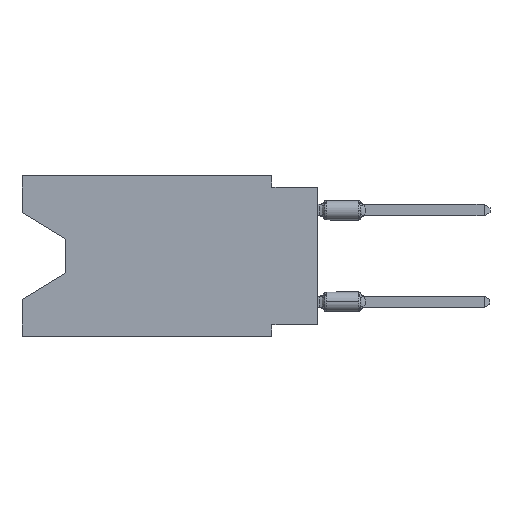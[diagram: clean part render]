
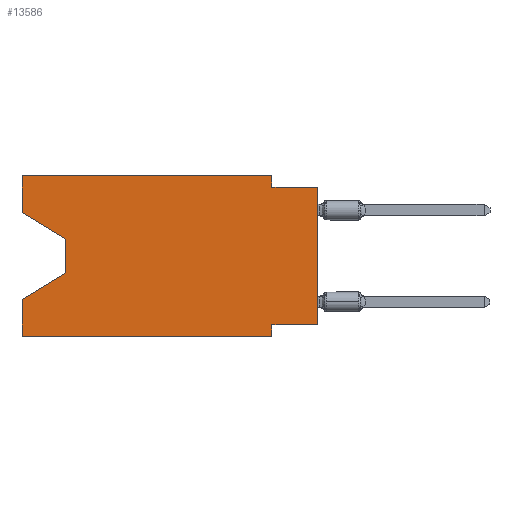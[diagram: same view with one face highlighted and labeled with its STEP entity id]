
A CAD part, left-side view. The second image highlights one B-rep face of the part: STEP entity #13586.
In plain terms, the highlighted planar face has unit normal (-1, 0, 0).
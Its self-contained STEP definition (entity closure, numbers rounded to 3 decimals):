
#43 = VERTEX_POINT ( 'NONE', #5842 ) ;
#48 = DIRECTION ( 'NONE',  ( 0., 0., 1. ) ) ;
#241 = CARTESIAN_POINT ( 'NONE',  ( 0., 2.54, -0.635 ) ) ;
#380 = VECTOR ( 'NONE', #11829, 1000. ) ;
#426 = CARTESIAN_POINT ( 'NONE',  ( 0., 0., -8.255 ) ) ;
#474 = EDGE_CURVE ( 'NONE', #11368, #16184, #8024, .T. ) ;
#653 = DIRECTION ( 'NONE',  ( 0., -1., 0. ) ) ;
#946 = CARTESIAN_POINT ( 'NONE',  ( 0., 2.54, -8.255 ) ) ;
#982 = CARTESIAN_POINT ( 'NONE',  ( 0., 16.383, 0. ) ) ;
#1346 = PLANE ( 'NONE',  #4279 ) ;
#1744 = LINE ( 'NONE', #7595, #12740 ) ;
#1861 = CARTESIAN_POINT ( 'NONE',  ( 0., 16.383, -8.89 ) ) ;
#1986 = LINE ( 'NONE', #13140, #380 ) ;
#2084 = DIRECTION ( 'NONE',  ( 0., 0., 1. ) ) ;
#2108 = CARTESIAN_POINT ( 'NONE',  ( 0., 2.54, 0. ) ) ;
#2224 = CARTESIAN_POINT ( 'NONE',  ( 0., 16.383, -8.89 ) ) ;
#2281 = VECTOR ( 'NONE', #18322, 1000. ) ;
#2501 = ORIENTED_EDGE ( 'NONE', *, *, #15400, .F. ) ;
#2663 = VERTEX_POINT ( 'NONE', #426 ) ;
#2858 = VECTOR ( 'NONE', #16302, 1000. ) ;
#2862 = EDGE_CURVE ( 'NONE', #5707, #16420, #9345, .T. ) ;
#2960 = CARTESIAN_POINT ( 'NONE',  ( 0., 16.383, -2.038 ) ) ;
#3248 = EDGE_CURVE ( 'NONE', #10550, #15878, #7563, .T. ) ;
#3447 = VERTEX_POINT ( 'NONE', #17375 ) ;
#3516 = VECTOR ( 'NONE', #48, 1000. ) ;
#3518 = CARTESIAN_POINT ( 'NONE',  ( 0., 13.97, -3.505 ) ) ;
#3619 = ORIENTED_EDGE ( 'NONE', *, *, #9178, .T. ) ;
#4067 = CARTESIAN_POINT ( 'NONE',  ( 0., 13.97, -3.505 ) ) ;
#4155 = ORIENTED_EDGE ( 'NONE', *, *, #17884, .T. ) ;
#4279 = AXIS2_PLACEMENT_3D ( 'NONE', #12594, #7189, #7271 ) ;
#4554 = DIRECTION ( 'NONE',  ( 0., -1., 0. ) ) ;
#4651 = CARTESIAN_POINT ( 'NONE',  ( 0., 16.383, 0. ) ) ;
#4839 = LINE ( 'NONE', #4651, #13966 ) ;
#5613 = VERTEX_POINT ( 'NONE', #12944 ) ;
#5678 = CARTESIAN_POINT ( 'NONE',  ( 0., 13.97, -5.385 ) ) ;
#5707 = VERTEX_POINT ( 'NONE', #10988 ) ;
#5842 = CARTESIAN_POINT ( 'NONE',  ( 0., 0., -0.635 ) ) ;
#6115 = VECTOR ( 'NONE', #8642, 1000. ) ;
#6698 = ORIENTED_EDGE ( 'NONE', *, *, #11343, .F. ) ;
#7189 = DIRECTION ( 'NONE',  ( 1., 0., 0. ) ) ;
#7271 = DIRECTION ( 'NONE',  ( 0., 0., -1. ) ) ;
#7288 = CARTESIAN_POINT ( 'NONE',  ( 0., 0., 0. ) ) ;
#7563 = LINE ( 'NONE', #17420, #17422 ) ;
#7582 = DIRECTION ( 'NONE',  ( 0., 0., -1. ) ) ;
#7595 = CARTESIAN_POINT ( 'NONE',  ( 0., 0., -0.635 ) ) ;
#7803 = ORIENTED_EDGE ( 'NONE', *, *, #15040, .F. ) ;
#8024 = LINE ( 'NONE', #13697, #2858 ) ;
#8642 = DIRECTION ( 'NONE',  ( 0., -0.855, -0.519 ) ) ;
#8944 = EDGE_LOOP ( 'NONE', ( #4155, #11613, #11654, #17715, #15608, #7803, #2501, #3619, #12137, #17951, #6698, #16190 ) ) ;
#9178 = EDGE_CURVE ( 'NONE', #2663, #43, #15581, .T. ) ;
#9345 = LINE ( 'NONE', #2108, #9988 ) ;
#9988 = VECTOR ( 'NONE', #7582, 1000. ) ;
#10150 = CARTESIAN_POINT ( 'NONE',  ( 0., 16.383, -6.852 ) ) ;
#10307 = LINE ( 'NONE', #10490, #12962 ) ;
#10490 = CARTESIAN_POINT ( 'NONE',  ( 0., 0., -8.255 ) ) ;
#10535 = EDGE_CURVE ( 'NONE', #16420, #43, #1744, .T. ) ;
#10550 = VERTEX_POINT ( 'NONE', #2960 ) ;
#10564 = LINE ( 'NONE', #3518, #14697 ) ;
#10988 = CARTESIAN_POINT ( 'NONE',  ( 0., 2.54, 0. ) ) ;
#11072 = LINE ( 'NONE', #5678, #2281 ) ;
#11343 = EDGE_CURVE ( 'NONE', #15878, #5707, #4839, .T. ) ;
#11368 = VERTEX_POINT ( 'NONE', #1861 ) ;
#11457 = VERTEX_POINT ( 'NONE', #946 ) ;
#11613 = ORIENTED_EDGE ( 'NONE', *, *, #14179, .T. ) ;
#11654 = ORIENTED_EDGE ( 'NONE', *, *, #17752, .T. ) ;
#11829 = DIRECTION ( 'NONE',  ( 0., 0., -1. ) ) ;
#12086 = VERTEX_POINT ( 'NONE', #4067 ) ;
#12137 = ORIENTED_EDGE ( 'NONE', *, *, #10535, .F. ) ;
#12594 = CARTESIAN_POINT ( 'NONE',  ( 0., 16.383, 0. ) ) ;
#12740 = VECTOR ( 'NONE', #17550, 1000. ) ;
#12825 = CARTESIAN_POINT ( 'NONE',  ( 0., 16.383, -2.038 ) ) ;
#12944 = CARTESIAN_POINT ( 'NONE',  ( 0., 2.54, -8.89 ) ) ;
#12962 = VECTOR ( 'NONE', #15989, 1000. ) ;
#13140 = CARTESIAN_POINT ( 'NONE',  ( 0., 2.54, -8.89 ) ) ;
#13586 = ADVANCED_FACE ( 'NONE', ( #14255 ), #1346, .F. ) ;
#13697 = CARTESIAN_POINT ( 'NONE',  ( 0., 16.383, 0. ) ) ;
#13966 = VECTOR ( 'NONE', #4554, 1000. ) ;
#14179 = EDGE_CURVE ( 'NONE', #12086, #3447, #10564, .T. ) ;
#14255 = FACE_OUTER_BOUND ( 'NONE', #8944, .T. ) ;
#14667 = DIRECTION ( 'NONE',  ( 0., 0., -1. ) ) ;
#14697 = VECTOR ( 'NONE', #14667, 1000. ) ;
#14959 = LINE ( 'NONE', #2224, #16938 ) ;
#15040 = EDGE_CURVE ( 'NONE', #11457, #5613, #1986, .T. ) ;
#15400 = EDGE_CURVE ( 'NONE', #2663, #11457, #10307, .T. ) ;
#15581 = LINE ( 'NONE', #7288, #3516 ) ;
#15608 = ORIENTED_EDGE ( 'NONE', *, *, #18023, .T. ) ;
#15805 = LINE ( 'NONE', #12825, #6115 ) ;
#15878 = VERTEX_POINT ( 'NONE', #982 ) ;
#15989 = DIRECTION ( 'NONE',  ( 0., 1., 0. ) ) ;
#16184 = VERTEX_POINT ( 'NONE', #10150 ) ;
#16190 = ORIENTED_EDGE ( 'NONE', *, *, #3248, .F. ) ;
#16302 = DIRECTION ( 'NONE',  ( 0., 0., 1. ) ) ;
#16420 = VERTEX_POINT ( 'NONE', #241 ) ;
#16938 = VECTOR ( 'NONE', #653, 1000. ) ;
#17375 = CARTESIAN_POINT ( 'NONE',  ( 0., 13.97, -5.385 ) ) ;
#17420 = CARTESIAN_POINT ( 'NONE',  ( 0., 16.383, 0. ) ) ;
#17422 = VECTOR ( 'NONE', #2084, 1000. ) ;
#17550 = DIRECTION ( 'NONE',  ( 0., -1., 0. ) ) ;
#17715 = ORIENTED_EDGE ( 'NONE', *, *, #474, .F. ) ;
#17752 = EDGE_CURVE ( 'NONE', #3447, #16184, #11072, .T. ) ;
#17884 = EDGE_CURVE ( 'NONE', #10550, #12086, #15805, .T. ) ;
#17951 = ORIENTED_EDGE ( 'NONE', *, *, #2862, .F. ) ;
#18023 = EDGE_CURVE ( 'NONE', #11368, #5613, #14959, .T. ) ;
#18322 = DIRECTION ( 'NONE',  ( 0., 0.855, -0.519 ) ) ;
